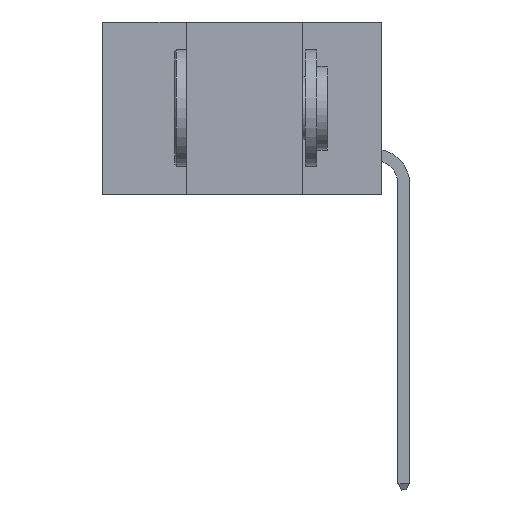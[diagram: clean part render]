
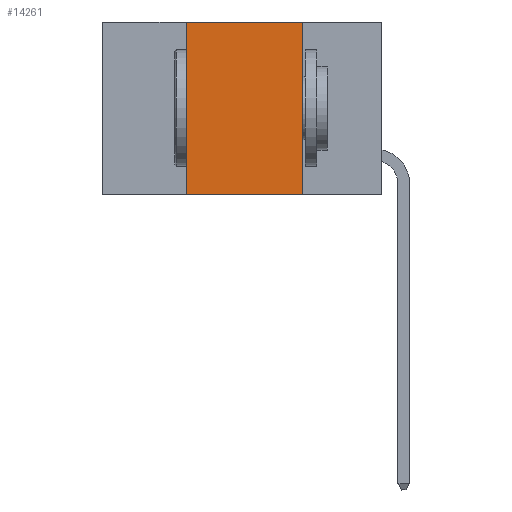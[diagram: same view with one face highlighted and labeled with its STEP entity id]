
A CAD part, left-side view. The second image highlights one B-rep face of the part: STEP entity #14261.
In plain terms, the highlighted planar face has unit normal (-1, 0, 0).
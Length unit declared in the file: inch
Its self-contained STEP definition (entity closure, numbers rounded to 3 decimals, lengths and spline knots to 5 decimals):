
#291 = DIRECTION ( 'NONE',  ( 0., 0., 1. ) ) ;
#890 = ORIENTED_EDGE ( 'NONE', *, *, #6115, .F. ) ;
#1320 = VERTEX_POINT ( 'NONE', #5600 ) ;
#1724 = CARTESIAN_POINT ( 'NONE',  ( 0., 0.42, 0. ) ) ;
#2200 = DIRECTION ( 'NONE',  ( 0., 0., -1. ) ) ;
#2279 = AXIS2_PLACEMENT_3D ( 'NONE', #17831, #5171, #2200 ) ;
#3182 = VERTEX_POINT ( 'NONE', #14061 ) ;
#3323 = FACE_OUTER_BOUND ( 'NONE', #19529, .T. ) ;
#3857 = CARTESIAN_POINT ( 'NONE',  ( 0., 0.17, 0. ) ) ;
#4129 = VECTOR ( 'NONE', #291, 39.37008 ) ;
#5171 = DIRECTION ( 'NONE',  ( 1., 0., 0. ) ) ;
#5600 = CARTESIAN_POINT ( 'NONE',  ( 0., 0.42, -0.37 ) ) ;
#5634 = CARTESIAN_POINT ( 'NONE',  ( 0., 0.17, -0.37 ) ) ;
#6115 = EDGE_CURVE ( 'NONE', #3182, #16871, #7145, .T. ) ;
#7065 = LINE ( 'NONE', #1724, #4129 ) ;
#7145 = LINE ( 'NONE', #3857, #9328 ) ;
#7597 = ORIENTED_EDGE ( 'NONE', *, *, #12567, .F. ) ;
#8051 = CARTESIAN_POINT ( 'NONE',  ( 0., 0.6, 0. ) ) ;
#8681 = ORIENTED_EDGE ( 'NONE', *, *, #16460, .F. ) ;
#9328 = VECTOR ( 'NONE', #11570, 39.37008 ) ;
#11570 = DIRECTION ( 'NONE',  ( 0., 0., -1. ) ) ;
#12026 = CARTESIAN_POINT ( 'NONE',  ( 0., 0.6, -0.37 ) ) ;
#12567 = EDGE_CURVE ( 'NONE', #1320, #18208, #7065, .T. ) ;
#14061 = CARTESIAN_POINT ( 'NONE',  ( 0., 0.17, 0. ) ) ;
#14241 = VECTOR ( 'NONE', #15992, 39.37008 ) ;
#14261 = ADVANCED_FACE ( 'NONE', ( #3323 ), #14486, .F. ) ;
#14486 = PLANE ( 'NONE',  #2279 ) ;
#14509 = EDGE_CURVE ( 'NONE', #1320, #16871, #14748, .T. ) ;
#14748 = LINE ( 'NONE', #12026, #18656 ) ;
#15045 = CARTESIAN_POINT ( 'NONE',  ( 0., 0.42, 0. ) ) ;
#15992 = DIRECTION ( 'NONE',  ( 0., -1., 0. ) ) ;
#16460 = EDGE_CURVE ( 'NONE', #18208, #3182, #18152, .T. ) ;
#16741 = DIRECTION ( 'NONE',  ( 0., -1., 0. ) ) ;
#16871 = VERTEX_POINT ( 'NONE', #5634 ) ;
#17831 = CARTESIAN_POINT ( 'NONE',  ( 0., 0.6, 0. ) ) ;
#18152 = LINE ( 'NONE', #8051, #14241 ) ;
#18203 = ORIENTED_EDGE ( 'NONE', *, *, #14509, .T. ) ;
#18208 = VERTEX_POINT ( 'NONE', #15045 ) ;
#18656 = VECTOR ( 'NONE', #16741, 39.37008 ) ;
#19529 = EDGE_LOOP ( 'NONE', ( #890, #8681, #7597, #18203 ) ) ;
